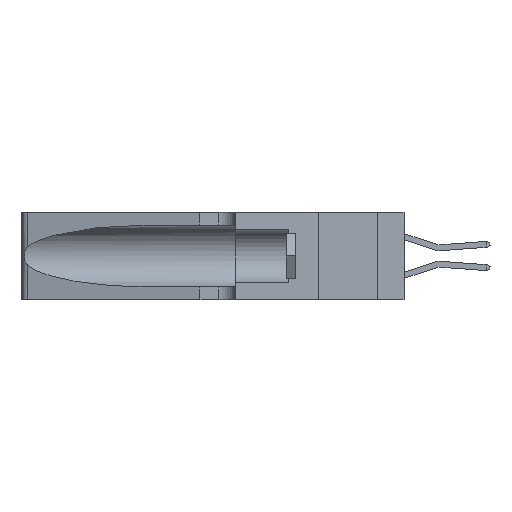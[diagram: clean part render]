
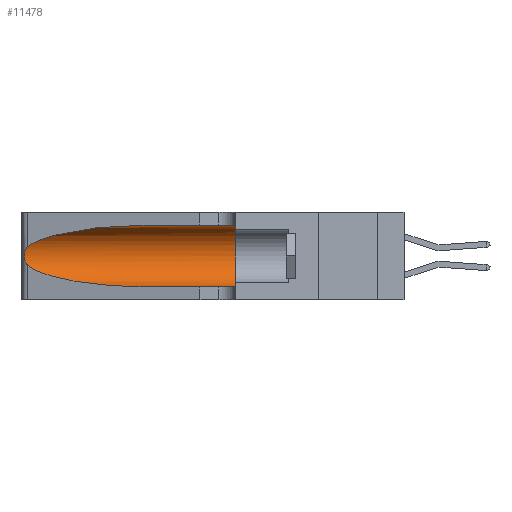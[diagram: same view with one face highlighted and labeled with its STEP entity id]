
A CAD part, left-side view. The second image highlights one B-rep face of the part: STEP entity #11478.
In plain terms, the highlighted cylindrical face has radius 3.308 mm (diameter 6.617 mm), a partial arc.
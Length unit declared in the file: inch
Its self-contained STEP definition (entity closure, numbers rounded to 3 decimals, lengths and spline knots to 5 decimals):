
#282 = CARTESIAN_POINT ( 'NONE',  ( 0.25487, 1.22718, 0.22369 ) ) ;
#369 = VERTEX_POINT ( 'NONE', #741 ) ;
#741 = CARTESIAN_POINT ( 'NONE',  ( 0.1305, 0.72297, 0.05475 ) ) ;
#1154 = EDGE_CURVE ( 'NONE', #369, #13773, #20293, .T. ) ;
#1268 = VERTEX_POINT ( 'NONE', #20289 ) ;
#1483 = CARTESIAN_POINT ( 'NONE',  ( 0.1305, 0.35, 0.185 ) ) ;
#1566 = EDGE_CURVE ( 'NONE', #15276, #3458, #4600, .T. ) ;
#1603 = DIRECTION ( 'NONE',  ( 0., 1., 0. ) ) ;
#1793 = CARTESIAN_POINT ( 'NONE',  ( 0.2373, 1.15595, 0.28018 ) ) ;
#1844 = CARTESIAN_POINT ( 'NONE',  ( 0.25487, 1.22718, 0.14631 ) ) ;
#2115 = DIRECTION ( 'NONE',  ( 0., -1., 0. ) ) ;
#2279 = EDGE_LOOP ( 'NONE', ( #19967, #14004, #15103, #10662, #14351, #13846 ) ) ;
#2856 =( BOUNDED_CURVE ( )  B_SPLINE_CURVE ( 3, ( #13003, #15905, #6401, #11493 ),
 .UNSPECIFIED., .F., .F. ) 
 B_SPLINE_CURVE_WITH_KNOTS ( ( 4, 4 ),
 ( 3.44316, 4.71239 ),
 .UNSPECIFIED. ) 
 CURVE ( )  GEOMETRIC_REPRESENTATION_ITEM ( )  RATIONAL_B_SPLINE_CURVE ( ( 1., 0.87, 0.87, 1. ) ) 
 REPRESENTATION_ITEM ( '' )  );
#3458 = VERTEX_POINT ( 'NONE', #9593 ) ;
#3889 = DIRECTION ( 'NONE',  ( 0., -1., 0. ) ) ;
#4235 = CARTESIAN_POINT ( 'NONE',  ( 0.25555, 1.22994, 0.2215 ) ) ;
#4414 = CARTESIAN_POINT ( 'NONE',  ( 0.25639, 1.23184, 0.21858 ) ) ;
#4600 =( BOUNDED_CURVE ( )  B_SPLINE_CURVE ( 3, ( #19221, #11398, #1793, #14657 ),
 .UNSPECIFIED., .F., .F. ) 
 B_SPLINE_CURVE_WITH_KNOTS ( ( 4, 4 ),
 ( 1.5708, 2.84003 ),
 .UNSPECIFIED. ) 
 CURVE ( )  GEOMETRIC_REPRESENTATION_ITEM ( )  RATIONAL_B_SPLINE_CURVE ( ( 1., 0.87, 0.87, 1. ) ) 
 REPRESENTATION_ITEM ( '' )  );
#4756 = VERTEX_POINT ( 'NONE', #1844 ) ;
#4846 = CARTESIAN_POINT ( 'NONE',  ( 0.1305, 0.72297, 0.31525 ) ) ;
#4956 = EDGE_CURVE ( 'NONE', #3458, #4756, #15083, .T. ) ;
#5043 = CARTESIAN_POINT ( 'NONE',  ( 0.25555, 1.22993, 0.14849 ) ) ;
#6099 = CARTESIAN_POINT ( 'NONE',  ( 0.25787, 1.23484, 0.2124 ) ) ;
#6401 = CARTESIAN_POINT ( 'NONE',  ( 0.18966, 0.96281, 0.05475 ) ) ;
#6443 = VECTOR ( 'NONE', #3889, 39.37008 ) ;
#6630 = CARTESIAN_POINT ( 'NONE',  ( 0.25487, 1.22718, 0.14631 ) ) ;
#7869 = FACE_OUTER_BOUND ( 'NONE', #2279, .T. ) ;
#8908 = DIRECTION ( 'NONE',  ( 0., 0., -1. ) ) ;
#9311 = CARTESIAN_POINT ( 'NONE',  ( 0.26018, 1.23835, 0.19895 ) ) ;
#9581 = CARTESIAN_POINT ( 'NONE',  ( 0.25856, 1.23593, 0.16098 ) ) ;
#9593 = CARTESIAN_POINT ( 'NONE',  ( 0.25487, 1.22718, 0.22369 ) ) ;
#9646 = CARTESIAN_POINT ( 'NONE',  ( 0.26075, 1.23896, 0.19203 ) ) ;
#10230 = CARTESIAN_POINT ( 'NONE',  ( 0.1305, 1.61858, 0.05475 ) ) ;
#10662 = ORIENTED_EDGE ( 'NONE', *, *, #1154, .T. ) ;
#10804 = VECTOR ( 'NONE', #2115, 39.37008 ) ;
#11089 = CARTESIAN_POINT ( 'NONE',  ( 0.26017, 1.23833, 0.17102 ) ) ;
#11198 = AXIS2_PLACEMENT_3D ( 'NONE', #1483, #1603, #12582 ) ;
#11398 = CARTESIAN_POINT ( 'NONE',  ( 0.18966, 0.96281, 0.31525 ) ) ;
#11478 = ADVANCED_FACE ( 'NONE', ( #7869 ), #19428, .F. ) ;
#11493 = CARTESIAN_POINT ( 'NONE',  ( 0.1305, 0.72297, 0.05475 ) ) ;
#11522 = CARTESIAN_POINT ( 'NONE',  ( 0.25639, 1.23186, 0.15144 ) ) ;
#12582 = DIRECTION ( 'NONE',  ( 0., 0., 1. ) ) ;
#12671 = AXIS2_PLACEMENT_3D ( 'NONE', #18054, #13388, #8908 ) ;
#13003 = CARTESIAN_POINT ( 'NONE',  ( 0.25487, 1.22718, 0.14631 ) ) ;
#13388 = DIRECTION ( 'NONE',  ( 0., -1., 0. ) ) ;
#13773 = VERTEX_POINT ( 'NONE', #16084 ) ;
#13846 = ORIENTED_EDGE ( 'NONE', *, *, #16196, .F. ) ;
#14004 = ORIENTED_EDGE ( 'NONE', *, *, #4956, .T. ) ;
#14351 = ORIENTED_EDGE ( 'NONE', *, *, #18649, .F. ) ;
#14657 = CARTESIAN_POINT ( 'NONE',  ( 0.25487, 1.22718, 0.22369 ) ) ;
#15083 = B_SPLINE_CURVE_WITH_KNOTS ( 'NONE', 3,
 ( #282, #4235, #4414, #6099, #17177, #9311, #9646, #16065, #11089, #9581, #15864, #11522, #5043, #6630 ),
 .UNSPECIFIED., .F., .F.,
 ( 4, 2, 2, 2, 2, 2, 4 ),
 ( 0., 0.00027, 0.00053, 0.00107, 0.0016, 0.00187, 0.00214 ),
 .UNSPECIFIED. ) ;
#15103 = ORIENTED_EDGE ( 'NONE', *, *, #17973, .T. ) ;
#15276 = VERTEX_POINT ( 'NONE', #4846 ) ;
#15864 = CARTESIAN_POINT ( 'NONE',  ( 0.25789, 1.23486, 0.15765 ) ) ;
#15905 = CARTESIAN_POINT ( 'NONE',  ( 0.2373, 1.15595, 0.08982 ) ) ;
#16065 = CARTESIAN_POINT ( 'NONE',  ( 0.26075, 1.23896, 0.178 ) ) ;
#16084 = CARTESIAN_POINT ( 'NONE',  ( 0.1305, 0.35, 0.05475 ) ) ;
#16196 = EDGE_CURVE ( 'NONE', #15276, #1268, #18913, .T. ) ;
#16788 = CIRCLE ( 'NONE', #11198, 0.13025 ) ;
#17177 = CARTESIAN_POINT ( 'NONE',  ( 0.25854, 1.2359, 0.20912 ) ) ;
#17973 = EDGE_CURVE ( 'NONE', #4756, #369, #2856, .T. ) ;
#18054 = CARTESIAN_POINT ( 'NONE',  ( 0.1305, 1.61858, 0.185 ) ) ;
#18649 = EDGE_CURVE ( 'NONE', #1268, #13773, #16788, .T. ) ;
#18913 = LINE ( 'NONE', #19682, #10804 ) ;
#19221 = CARTESIAN_POINT ( 'NONE',  ( 0.1305, 0.72297, 0.31525 ) ) ;
#19428 = CYLINDRICAL_SURFACE ( 'NONE', #12671, 0.13025 ) ;
#19682 = CARTESIAN_POINT ( 'NONE',  ( 0.1305, 1.61858, 0.31525 ) ) ;
#19967 = ORIENTED_EDGE ( 'NONE', *, *, #1566, .T. ) ;
#20289 = CARTESIAN_POINT ( 'NONE',  ( 0.1305, 0.35, 0.31525 ) ) ;
#20293 = LINE ( 'NONE', #10230, #6443 ) ;
